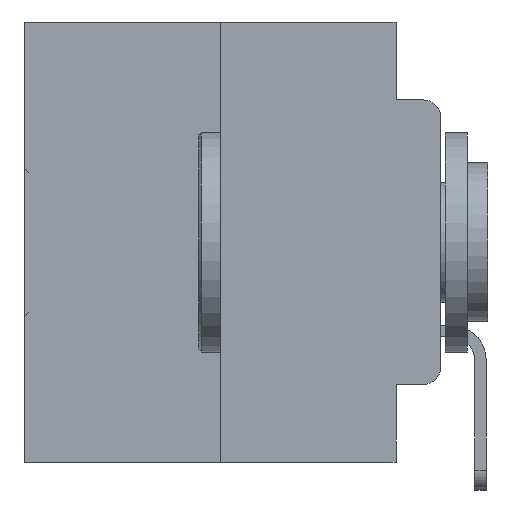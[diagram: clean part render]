
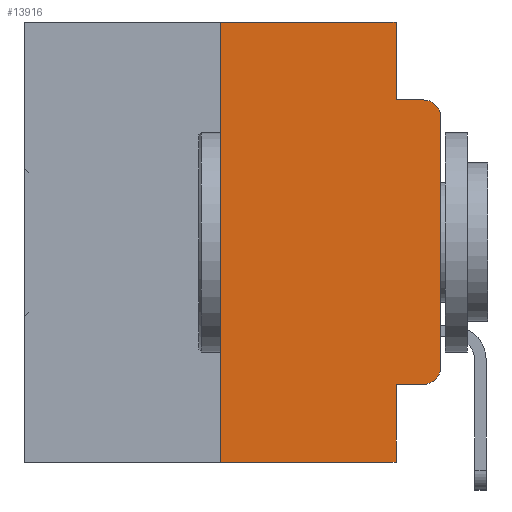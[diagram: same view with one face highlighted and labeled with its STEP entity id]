
A CAD part, left-side view. The second image highlights one B-rep face of the part: STEP entity #13916.
In plain terms, the highlighted planar face has unit normal (-1, 0, 0).
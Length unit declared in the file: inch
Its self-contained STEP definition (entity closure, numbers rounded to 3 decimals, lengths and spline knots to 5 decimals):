
#1000 = CARTESIAN_POINT ( 'NONE',  ( 0., 0.051, -0.4115 ) ) ;
#2130 = EDGE_CURVE ( 'NONE', #9436, #27541, #14271, .T. ) ;
#2421 = VECTOR ( 'NONE', #14064, 39.37008 ) ;
#2502 = CARTESIAN_POINT ( 'NONE',  ( 0., 0.051, -0.4115 ) ) ;
#2793 = CARTESIAN_POINT ( 'NONE',  ( 0., 0., -0.1085 ) ) ;
#3704 = DIRECTION ( 'NONE',  ( 0., 0., -1. ) ) ;
#3853 = ORIENTED_EDGE ( 'NONE', *, *, #20459, .F. ) ;
#5609 = ORIENTED_EDGE ( 'NONE', *, *, #14509, .F. ) ;
#6168 = CARTESIAN_POINT ( 'NONE',  ( 0., 0.051, 0. ) ) ;
#6587 = LINE ( 'NONE', #30312, #20910 ) ;
#7059 = DIRECTION ( 'NONE',  ( -1., 0., 0. ) ) ;
#7282 = ORIENTED_EDGE ( 'NONE', *, *, #21756, .T. ) ;
#7549 = DIRECTION ( 'NONE',  ( -1., 0., 0. ) ) ;
#7593 = VECTOR ( 'NONE', #3704, 39.37008 ) ;
#7672 = CARTESIAN_POINT ( 'NONE',  ( 0., 0.473, 0. ) ) ;
#8515 = ORIENTED_EDGE ( 'NONE', *, *, #13873, .T. ) ;
#8597 = CARTESIAN_POINT ( 'NONE',  ( 0., 0.25, 0. ) ) ;
#8714 = EDGE_CURVE ( 'NONE', #26750, #29663, #22845, .T. ) ;
#9390 = VECTOR ( 'NONE', #10324, 39.37008 ) ;
#9436 = VERTEX_POINT ( 'NONE', #1000 ) ;
#9806 = VERTEX_POINT ( 'NONE', #2793 ) ;
#10099 = ORIENTED_EDGE ( 'NONE', *, *, #8714, .F. ) ;
#10200 = LINE ( 'NONE', #29804, #9390 ) ;
#10324 = DIRECTION ( 'NONE',  ( 0., 0., 1. ) ) ;
#10762 = AXIS2_PLACEMENT_3D ( 'NONE', #22589, #7549, #25061 ) ;
#10890 = LINE ( 'NONE', #2502, #23361 ) ;
#11051 = CARTESIAN_POINT ( 'NONE',  ( 0., 0.25, -0.5 ) ) ;
#11487 = CARTESIAN_POINT ( 'NONE',  ( 0., 0.051, -0.0885 ) ) ;
#11678 = CARTESIAN_POINT ( 'NONE',  ( 0., 0.02, -0.4115 ) ) ;
#12008 = CARTESIAN_POINT ( 'NONE',  ( 0., 0.051, -0.0885 ) ) ;
#12664 = VECTOR ( 'NONE', #24776, 39.37008 ) ;
#12728 = PLANE ( 'NONE',  #20876 ) ;
#13346 = ORIENTED_EDGE ( 'NONE', *, *, #15184, .T. ) ;
#13873 = EDGE_CURVE ( 'NONE', #9806, #29663, #22371, .T. ) ;
#13916 = ADVANCED_FACE ( 'NONE', ( #15050 ), #12728, .F. ) ;
#14064 = DIRECTION ( 'NONE',  ( 0., -1., 0. ) ) ;
#14271 = LINE ( 'NONE', #27130, #12664 ) ;
#14283 = CARTESIAN_POINT ( 'NONE',  ( 0., 0.051, 0. ) ) ;
#14509 = EDGE_CURVE ( 'NONE', #18199, #20766, #10200, .T. ) ;
#14540 = CARTESIAN_POINT ( 'NONE',  ( 0., 0.051, -0.5 ) ) ;
#15050 = FACE_OUTER_BOUND ( 'NONE', #31594, .T. ) ;
#15105 = DIRECTION ( 'NONE',  ( 0., -1., 0. ) ) ;
#15184 = EDGE_CURVE ( 'NONE', #18199, #27541, #22284, .T. ) ;
#15392 = DIRECTION ( 'NONE',  ( 0., 0., -1. ) ) ;
#15570 = EDGE_CURVE ( 'NONE', #23382, #9806, #6587, .T. ) ;
#15571 = DIRECTION ( 'NONE',  ( 0., -1., 0. ) ) ;
#15719 = ORIENTED_EDGE ( 'NONE', *, *, #18465, .T. ) ;
#16866 = ORIENTED_EDGE ( 'NONE', *, *, #30698, .F. ) ;
#17434 = CARTESIAN_POINT ( 'NONE',  ( 0., 0., -0.3915 ) ) ;
#18199 = VERTEX_POINT ( 'NONE', #11051 ) ;
#18381 = DIRECTION ( 'NONE',  ( 0., 0., 1. ) ) ;
#18465 = EDGE_CURVE ( 'NONE', #25548, #23382, #26390, .T. ) ;
#19500 = DIRECTION ( 'NONE',  ( 0., -1., 0. ) ) ;
#20391 = VECTOR ( 'NONE', #15105, 39.37008 ) ;
#20459 = EDGE_CURVE ( 'NONE', #20766, #29889, #26778, .T. ) ;
#20766 = VERTEX_POINT ( 'NONE', #8597 ) ;
#20775 = CARTESIAN_POINT ( 'NONE',  ( 0., 0.02, -0.0885 ) ) ;
#20817 = VECTOR ( 'NONE', #19500, 39.37008 ) ;
#20876 = AXIS2_PLACEMENT_3D ( 'NONE', #7672, #29846, #15392 ) ;
#20910 = VECTOR ( 'NONE', #18381, 39.37008 ) ;
#21140 = ORIENTED_EDGE ( 'NONE', *, *, #15570, .T. ) ;
#21756 = EDGE_CURVE ( 'NONE', #9436, #25548, #10890, .T. ) ;
#22169 = CARTESIAN_POINT ( 'NONE',  ( 0., 0.02, -0.3915 ) ) ;
#22284 = LINE ( 'NONE', #26766, #20817 ) ;
#22371 = CIRCLE ( 'NONE', #10762, 0.02 ) ;
#22589 = CARTESIAN_POINT ( 'NONE',  ( 0., 0.02, -0.1085 ) ) ;
#22845 = LINE ( 'NONE', #11487, #2421 ) ;
#23361 = VECTOR ( 'NONE', #15571, 39.37008 ) ;
#23382 = VERTEX_POINT ( 'NONE', #17434 ) ;
#24620 = DIRECTION ( 'NONE',  ( 0., 0., -1. ) ) ;
#24776 = DIRECTION ( 'NONE',  ( 0., 0., -1. ) ) ;
#25061 = DIRECTION ( 'NONE',  ( 0., 0., -1. ) ) ;
#25548 = VERTEX_POINT ( 'NONE', #11678 ) ;
#25762 = AXIS2_PLACEMENT_3D ( 'NONE', #22169, #7059, #24620 ) ;
#26390 = CIRCLE ( 'NONE', #25762, 0.02 ) ;
#26399 = ORIENTED_EDGE ( 'NONE', *, *, #2130, .F. ) ;
#26750 = VERTEX_POINT ( 'NONE', #12008 ) ;
#26766 = CARTESIAN_POINT ( 'NONE',  ( 0., 0.473, -0.5 ) ) ;
#26778 = LINE ( 'NONE', #29579, #20391 ) ;
#27130 = CARTESIAN_POINT ( 'NONE',  ( 0., 0.051, 0. ) ) ;
#27394 = LINE ( 'NONE', #14283, #7593 ) ;
#27541 = VERTEX_POINT ( 'NONE', #14540 ) ;
#29579 = CARTESIAN_POINT ( 'NONE',  ( 0., 0.473, 0. ) ) ;
#29663 = VERTEX_POINT ( 'NONE', #20775 ) ;
#29804 = CARTESIAN_POINT ( 'NONE',  ( 0., 0.25, 0. ) ) ;
#29846 = DIRECTION ( 'NONE',  ( 1., 0., 0. ) ) ;
#29889 = VERTEX_POINT ( 'NONE', #6168 ) ;
#30312 = CARTESIAN_POINT ( 'NONE',  ( 0., 0., 0. ) ) ;
#30698 = EDGE_CURVE ( 'NONE', #29889, #26750, #27394, .T. ) ;
#31594 = EDGE_LOOP ( 'NONE', ( #21140, #8515, #10099, #16866, #3853, #5609, #13346, #26399, #7282, #15719 ) ) ;
